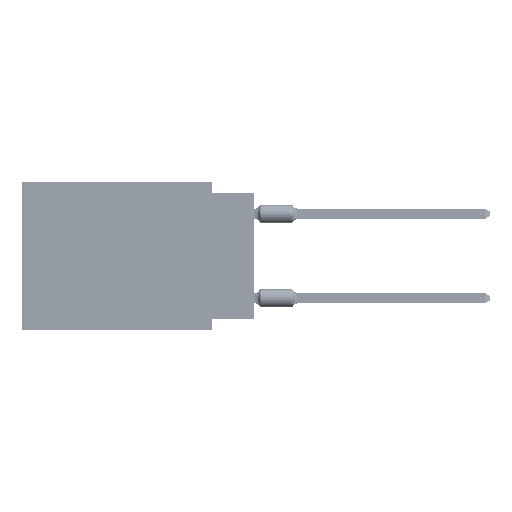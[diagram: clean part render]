
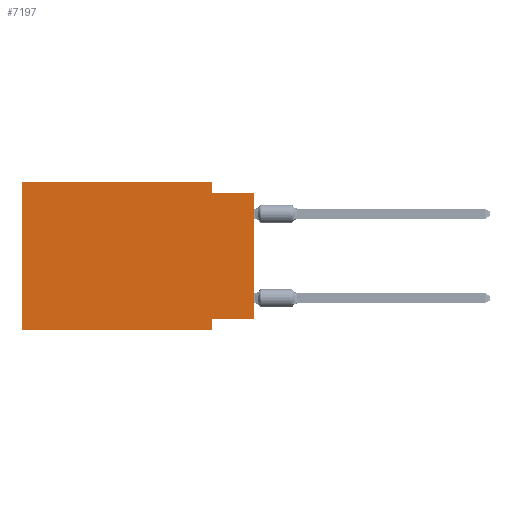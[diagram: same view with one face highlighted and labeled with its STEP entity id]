
A CAD part, left-side view. The second image highlights one B-rep face of the part: STEP entity #7197.
In plain terms, the highlighted planar face has unit normal (-1, 0, 0).
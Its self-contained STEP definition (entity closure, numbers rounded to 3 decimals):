
#635 = CARTESIAN_POINT ( 'NONE',  ( 0., 0., -8.255 ) ) ;
#1158 = DIRECTION ( 'NONE',  ( 0., 0., -1. ) ) ;
#4234 = VECTOR ( 'NONE', #44935, 1000. ) ;
#4422 = EDGE_CURVE ( 'NONE', #48584, #50517, #46024, .T. ) ;
#5073 = DIRECTION ( 'NONE',  ( 0., -1., 0. ) ) ;
#6517 = LINE ( 'NONE', #7239, #69446 ) ;
#6594 = CARTESIAN_POINT ( 'NONE',  ( 0., 2.54, -8.89 ) ) ;
#7197 = ADVANCED_FACE ( 'NONE', ( #38311 ), #60107, .F. ) ;
#7239 = CARTESIAN_POINT ( 'NONE',  ( 0., 2.54, 0. ) ) ;
#8314 = DIRECTION ( 'NONE',  ( 0., 1., 0. ) ) ;
#8510 = VECTOR ( 'NONE', #61527, 1000. ) ;
#11130 = CARTESIAN_POINT ( 'NONE',  ( 0., 13.97, 0. ) ) ;
#11929 = ORIENTED_EDGE ( 'NONE', *, *, #46173, .T. ) ;
#12924 = ORIENTED_EDGE ( 'NONE', *, *, #61100, .F. ) ;
#13641 = VECTOR ( 'NONE', #5073, 1000. ) ;
#13887 = CARTESIAN_POINT ( 'NONE',  ( 0., 13.97, 0. ) ) ;
#14093 = VERTEX_POINT ( 'NONE', #65912 ) ;
#14124 = ORIENTED_EDGE ( 'NONE', *, *, #48393, .F. ) ;
#16155 = CARTESIAN_POINT ( 'NONE',  ( 0., 13.97, -8.89 ) ) ;
#16667 = EDGE_CURVE ( 'NONE', #48410, #30247, #23422, .T. ) ;
#18331 = CARTESIAN_POINT ( 'NONE',  ( 0., 0., -8.255 ) ) ;
#23140 = LINE ( 'NONE', #62424, #4234 ) ;
#23422 = LINE ( 'NONE', #39025, #8510 ) ;
#23970 = EDGE_CURVE ( 'NONE', #30247, #14093, #34634, .T. ) ;
#24226 = DIRECTION ( 'NONE',  ( 0., -1., 0. ) ) ;
#24694 = ORIENTED_EDGE ( 'NONE', *, *, #67660, .F. ) ;
#24775 = ORIENTED_EDGE ( 'NONE', *, *, #23970, .F. ) ;
#27046 = ORIENTED_EDGE ( 'NONE', *, *, #16667, .F. ) ;
#27597 = DIRECTION ( 'NONE',  ( 1., 0., 0. ) ) ;
#29611 = DIRECTION ( 'NONE',  ( 0., -1., 0. ) ) ;
#29870 = AXIS2_PLACEMENT_3D ( 'NONE', #11130, #27597, #65828 ) ;
#30247 = VERTEX_POINT ( 'NONE', #63950 ) ;
#34427 = ORIENTED_EDGE ( 'NONE', *, *, #4422, .F. ) ;
#34512 = VECTOR ( 'NONE', #8314, 1000. ) ;
#34634 = LINE ( 'NONE', #13887, #41631 ) ;
#36560 = LINE ( 'NONE', #58384, #64746 ) ;
#37252 = DIRECTION ( 'NONE',  ( 0., 0., 1. ) ) ;
#38311 = FACE_OUTER_BOUND ( 'NONE', #58897, .T. ) ;
#39025 = CARTESIAN_POINT ( 'NONE',  ( 0., 13.97, 0. ) ) ;
#39768 = LINE ( 'NONE', #18331, #34512 ) ;
#40281 = VECTOR ( 'NONE', #24226, 1000. ) ;
#41631 = VECTOR ( 'NONE', #29611, 1000. ) ;
#42789 = CARTESIAN_POINT ( 'NONE',  ( 0., 0., -0.635 ) ) ;
#43302 = LINE ( 'NONE', #16155, #13641 ) ;
#44935 = DIRECTION ( 'NONE',  ( 0., 0., -1. ) ) ;
#46024 = LINE ( 'NONE', #61392, #40281 ) ;
#46173 = EDGE_CURVE ( 'NONE', #48410, #60736, #43302, .T. ) ;
#48393 = EDGE_CURVE ( 'NONE', #64235, #60736, #23140, .T. ) ;
#48410 = VERTEX_POINT ( 'NONE', #56009 ) ;
#48568 = CARTESIAN_POINT ( 'NONE',  ( 0., 2.54, -8.255 ) ) ;
#48584 = VERTEX_POINT ( 'NONE', #60208 ) ;
#50517 = VERTEX_POINT ( 'NONE', #42789 ) ;
#56009 = CARTESIAN_POINT ( 'NONE',  ( 0., 13.97, -8.89 ) ) ;
#58384 = CARTESIAN_POINT ( 'NONE',  ( 0., 0., 0. ) ) ;
#58897 = EDGE_LOOP ( 'NONE', ( #63676, #34427, #12924, #24775, #27046, #11929, #14124, #24694 ) ) ;
#60107 = PLANE ( 'NONE',  #29870 ) ;
#60208 = CARTESIAN_POINT ( 'NONE',  ( 0., 2.54, -0.635 ) ) ;
#60736 = VERTEX_POINT ( 'NONE', #6594 ) ;
#61100 = EDGE_CURVE ( 'NONE', #14093, #48584, #6517, .T. ) ;
#61392 = CARTESIAN_POINT ( 'NONE',  ( 0., 0., -0.635 ) ) ;
#61527 = DIRECTION ( 'NONE',  ( 0., 0., 1. ) ) ;
#61970 = VERTEX_POINT ( 'NONE', #635 ) ;
#62424 = CARTESIAN_POINT ( 'NONE',  ( 0., 2.54, -8.89 ) ) ;
#63676 = ORIENTED_EDGE ( 'NONE', *, *, #69631, .T. ) ;
#63950 = CARTESIAN_POINT ( 'NONE',  ( 0., 13.97, 0. ) ) ;
#64235 = VERTEX_POINT ( 'NONE', #48568 ) ;
#64746 = VECTOR ( 'NONE', #37252, 1000. ) ;
#65828 = DIRECTION ( 'NONE',  ( 0., 0., -1. ) ) ;
#65912 = CARTESIAN_POINT ( 'NONE',  ( 0., 2.54, 0. ) ) ;
#67660 = EDGE_CURVE ( 'NONE', #61970, #64235, #39768, .T. ) ;
#69446 = VECTOR ( 'NONE', #1158, 1000. ) ;
#69631 = EDGE_CURVE ( 'NONE', #61970, #50517, #36560, .T. ) ;
